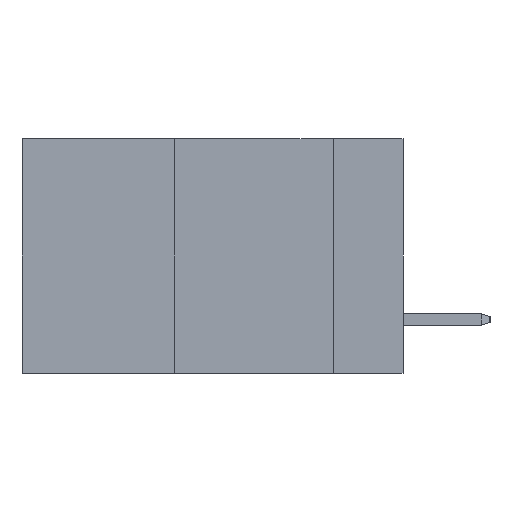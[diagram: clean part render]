
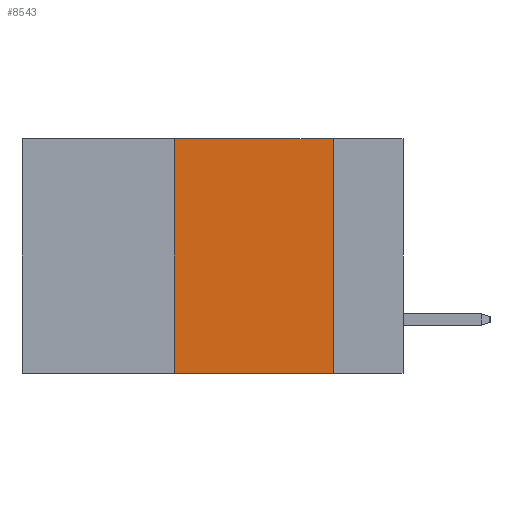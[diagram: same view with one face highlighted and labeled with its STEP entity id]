
A CAD part, left-side view. The second image highlights one B-rep face of the part: STEP entity #8543.
In plain terms, the highlighted planar face has unit normal (-1, 0, 0).
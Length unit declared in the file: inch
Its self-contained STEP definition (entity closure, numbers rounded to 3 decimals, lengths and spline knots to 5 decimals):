
#664 = CARTESIAN_POINT ( 'NONE',  ( 0., 0.6, -0.37 ) ) ;
#789 = DIRECTION ( 'NONE',  ( 1., 0., 0. ) ) ;
#1256 = CARTESIAN_POINT ( 'NONE',  ( 0., 0.11, 0. ) ) ;
#1273 = EDGE_CURVE ( 'NONE', #8787, #5309, #5762, .T. ) ;
#1331 = CARTESIAN_POINT ( 'NONE',  ( 0., 0.11, -0.37 ) ) ;
#1499 = VERTEX_POINT ( 'NONE', #1331 ) ;
#1502 = DIRECTION ( 'NONE',  ( 0., -1., 0. ) ) ;
#1528 = DIRECTION ( 'NONE',  ( 0., 0., 1. ) ) ;
#1533 = DIRECTION ( 'NONE',  ( 0., -1., 0. ) ) ;
#1986 = CARTESIAN_POINT ( 'NONE',  ( 0., 0.36, -0.37 ) ) ;
#2381 = CARTESIAN_POINT ( 'NONE',  ( 0., 0.6, 0. ) ) ;
#2898 = DIRECTION ( 'NONE',  ( 0., 0., -1. ) ) ;
#3181 = EDGE_CURVE ( 'NONE', #10996, #1499, #8236, .T. ) ;
#3415 = ORIENTED_EDGE ( 'NONE', *, *, #3847, .T. ) ;
#3847 = EDGE_CURVE ( 'NONE', #8787, #1499, #11379, .T. ) ;
#3871 = AXIS2_PLACEMENT_3D ( 'NONE', #9713, #789, #7684 ) ;
#4498 = VECTOR ( 'NONE', #1528, 39.37008 ) ;
#4832 = CARTESIAN_POINT ( 'NONE',  ( 0., 0.36, 0. ) ) ;
#5244 = PLANE ( 'NONE',  #3871 ) ;
#5309 = VERTEX_POINT ( 'NONE', #10273 ) ;
#5762 = LINE ( 'NONE', #4832, #4498 ) ;
#5976 = EDGE_CURVE ( 'NONE', #5309, #10996, #10316, .T. ) ;
#6241 = VECTOR ( 'NONE', #1533, 39.37008 ) ;
#6437 = ORIENTED_EDGE ( 'NONE', *, *, #1273, .F. ) ;
#7324 = VECTOR ( 'NONE', #2898, 39.37008 ) ;
#7502 = CARTESIAN_POINT ( 'NONE',  ( 0., 0.11, 0. ) ) ;
#7684 = DIRECTION ( 'NONE',  ( 0., 0., -1. ) ) ;
#7925 = FACE_OUTER_BOUND ( 'NONE', #9816, .T. ) ;
#8236 = LINE ( 'NONE', #1256, #7324 ) ;
#8543 = ADVANCED_FACE ( 'NONE', ( #7925 ), #5244, .F. ) ;
#8787 = VERTEX_POINT ( 'NONE', #1986 ) ;
#9406 = ORIENTED_EDGE ( 'NONE', *, *, #5976, .F. ) ;
#9713 = CARTESIAN_POINT ( 'NONE',  ( 0., 0.6, 0. ) ) ;
#9816 = EDGE_LOOP ( 'NONE', ( #9955, #9406, #6437, #3415 ) ) ;
#9955 = ORIENTED_EDGE ( 'NONE', *, *, #3181, .F. ) ;
#10169 = VECTOR ( 'NONE', #1502, 39.37008 ) ;
#10273 = CARTESIAN_POINT ( 'NONE',  ( 0., 0.36, 0. ) ) ;
#10316 = LINE ( 'NONE', #2381, #10169 ) ;
#10996 = VERTEX_POINT ( 'NONE', #7502 ) ;
#11379 = LINE ( 'NONE', #664, #6241 ) ;
